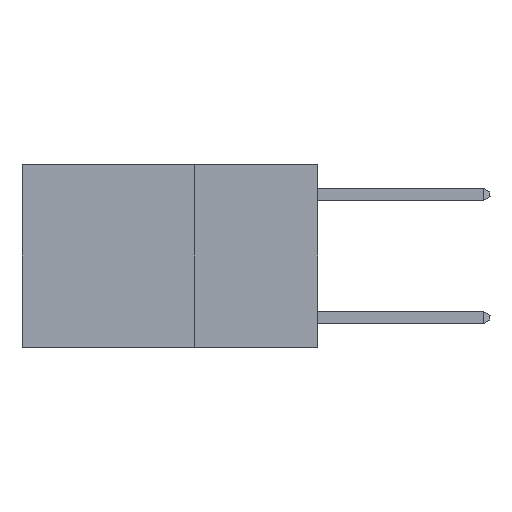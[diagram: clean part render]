
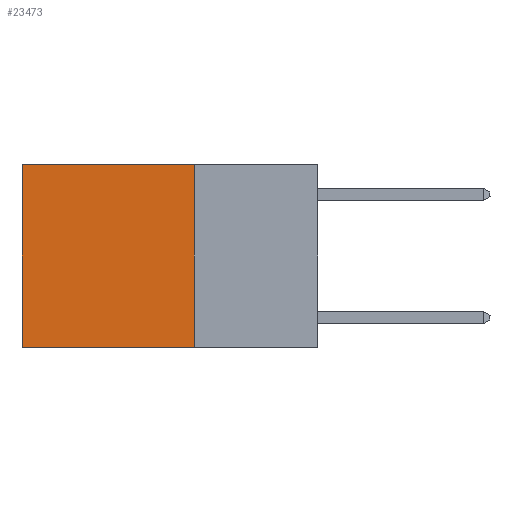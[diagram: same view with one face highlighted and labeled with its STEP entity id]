
A CAD part, left-side view. The second image highlights one B-rep face of the part: STEP entity #23473.
In plain terms, the highlighted planar face has unit normal (-1, 0, 0).
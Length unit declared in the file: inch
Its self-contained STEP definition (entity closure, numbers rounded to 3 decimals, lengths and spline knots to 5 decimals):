
#485 = VECTOR ( 'NONE', #3605, 39.37008 ) ;
#800 = ORIENTED_EDGE ( 'NONE', *, *, #16280, .T. ) ;
#1552 = PLANE ( 'NONE',  #23468 ) ;
#1650 = CARTESIAN_POINT ( 'NONE',  ( 0.2625, 0.6, 0. ) ) ;
#1843 = DIRECTION ( 'NONE',  ( 0., 0., -1. ) ) ;
#2764 = CARTESIAN_POINT ( 'NONE',  ( 0.2625, 0.25, 0. ) ) ;
#3605 = DIRECTION ( 'NONE',  ( 0., 1., 0. ) ) ;
#3689 = DIRECTION ( 'NONE',  ( 0., 1., 0. ) ) ;
#4543 = LINE ( 'NONE', #2764, #15679 ) ;
#5709 = VECTOR ( 'NONE', #7771, 39.37008 ) ;
#5964 = CARTESIAN_POINT ( 'NONE',  ( 0.2625, 0.25, 0. ) ) ;
#6169 = VERTEX_POINT ( 'NONE', #27284 ) ;
#7208 = VECTOR ( 'NONE', #3689, 39.37008 ) ;
#7771 = DIRECTION ( 'NONE',  ( 0., 0., -1. ) ) ;
#8013 = CARTESIAN_POINT ( 'NONE',  ( 0.2625, 0.25, 0. ) ) ;
#8960 = LINE ( 'NONE', #25751, #7208 ) ;
#9975 = LINE ( 'NONE', #27909, #5709 ) ;
#10405 = CARTESIAN_POINT ( 'NONE',  ( 0.2625, 0.25, 0. ) ) ;
#10678 = FACE_OUTER_BOUND ( 'NONE', #21825, .T. ) ;
#12222 = VERTEX_POINT ( 'NONE', #10405 ) ;
#13031 = ORIENTED_EDGE ( 'NONE', *, *, #17694, .F. ) ;
#13503 = DIRECTION ( 'NONE',  ( 0., 0., -1. ) ) ;
#14293 = VERTEX_POINT ( 'NONE', #20061 ) ;
#15111 = ORIENTED_EDGE ( 'NONE', *, *, #17914, .F. ) ;
#15679 = VECTOR ( 'NONE', #13503, 39.37008 ) ;
#16280 = EDGE_CURVE ( 'NONE', #21898, #6169, #9975, .T. ) ;
#17694 = EDGE_CURVE ( 'NONE', #14293, #6169, #8960, .T. ) ;
#17914 = EDGE_CURVE ( 'NONE', #12222, #14293, #4543, .T. ) ;
#19725 = EDGE_CURVE ( 'NONE', #12222, #21898, #28156, .T. ) ;
#20061 = CARTESIAN_POINT ( 'NONE',  ( 0.2625, 0.25, -0.37 ) ) ;
#20070 = DIRECTION ( 'NONE',  ( 1., 0., 0. ) ) ;
#21825 = EDGE_LOOP ( 'NONE', ( #800, #13031, #15111, #28023 ) ) ;
#21898 = VERTEX_POINT ( 'NONE', #1650 ) ;
#23468 = AXIS2_PLACEMENT_3D ( 'NONE', #5964, #20070, #1843 ) ;
#23473 = ADVANCED_FACE ( 'NONE', ( #10678 ), #1552, .F. ) ;
#25751 = CARTESIAN_POINT ( 'NONE',  ( 0.2625, 0.25, -0.37 ) ) ;
#27284 = CARTESIAN_POINT ( 'NONE',  ( 0.2625, 0.6, -0.37 ) ) ;
#27909 = CARTESIAN_POINT ( 'NONE',  ( 0.2625, 0.6, 0. ) ) ;
#28023 = ORIENTED_EDGE ( 'NONE', *, *, #19725, .T. ) ;
#28156 = LINE ( 'NONE', #8013, #485 ) ;
